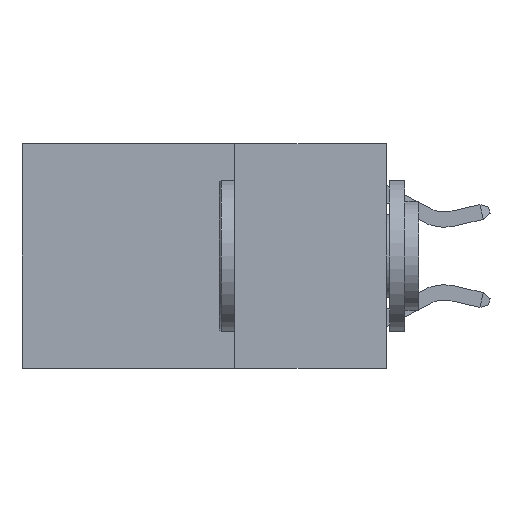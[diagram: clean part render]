
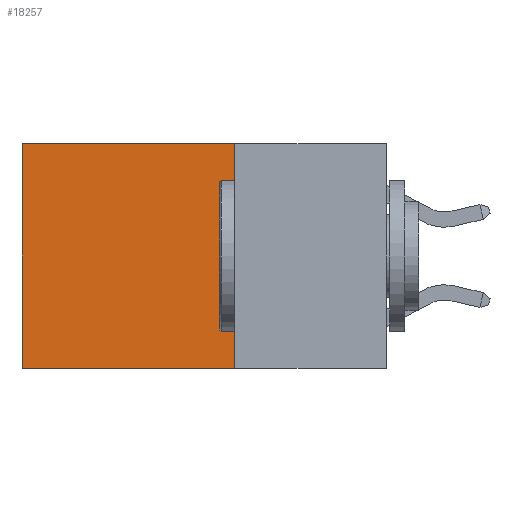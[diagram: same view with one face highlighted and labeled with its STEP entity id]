
A CAD part, left-side view. The second image highlights one B-rep face of the part: STEP entity #18257.
In plain terms, the highlighted planar face has unit normal (-1, 0, 0).
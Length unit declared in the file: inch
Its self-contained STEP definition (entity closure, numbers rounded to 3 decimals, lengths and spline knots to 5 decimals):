
#292 = CARTESIAN_POINT ( 'NONE',  ( 0.2625, 0.6, 0. ) ) ;
#810 = VERTEX_POINT ( 'NONE', #22380 ) ;
#1806 = EDGE_CURVE ( 'NONE', #18598, #12141, #10432, .T. ) ;
#2282 = LINE ( 'NONE', #292, #22768 ) ;
#3551 = DIRECTION ( 'NONE',  ( 0., 0., -1. ) ) ;
#5130 = VECTOR ( 'NONE', #16532, 39.37008 ) ;
#5199 = AXIS2_PLACEMENT_3D ( 'NONE', #7918, #26046, #3551 ) ;
#6414 = CARTESIAN_POINT ( 'NONE',  ( 0.2625, 0.6, -0.37 ) ) ;
#6752 = EDGE_CURVE ( 'NONE', #12141, #24361, #2282, .T. ) ;
#7513 = FACE_OUTER_BOUND ( 'NONE', #9814, .T. ) ;
#7712 = CARTESIAN_POINT ( 'NONE',  ( 0.2625, 0.25, 0. ) ) ;
#7918 = CARTESIAN_POINT ( 'NONE',  ( 0.2625, 0.25, 0. ) ) ;
#7941 = ORIENTED_EDGE ( 'NONE', *, *, #17400, .F. ) ;
#9814 = EDGE_LOOP ( 'NONE', ( #18756, #7941, #14336, #16081 ) ) ;
#10432 = LINE ( 'NONE', #12653, #19059 ) ;
#10559 = DIRECTION ( 'NONE',  ( 0., 1., 0. ) ) ;
#11722 = CARTESIAN_POINT ( 'NONE',  ( 0.2625, 0.25, 0. ) ) ;
#12141 = VERTEX_POINT ( 'NONE', #24973 ) ;
#12495 = VECTOR ( 'NONE', #13647, 39.37008 ) ;
#12570 = CARTESIAN_POINT ( 'NONE',  ( 0.2625, 0.25, -0.37 ) ) ;
#12653 = CARTESIAN_POINT ( 'NONE',  ( 0.2625, 0.25, 0. ) ) ;
#12789 = EDGE_CURVE ( 'NONE', #18598, #810, #16146, .T. ) ;
#13647 = DIRECTION ( 'NONE',  ( 0., 0., -1. ) ) ;
#14336 = ORIENTED_EDGE ( 'NONE', *, *, #12789, .F. ) ;
#16081 = ORIENTED_EDGE ( 'NONE', *, *, #1806, .T. ) ;
#16146 = LINE ( 'NONE', #7712, #12495 ) ;
#16532 = DIRECTION ( 'NONE',  ( 0., 1., 0. ) ) ;
#17400 = EDGE_CURVE ( 'NONE', #810, #24361, #24792, .T. ) ;
#18257 = ADVANCED_FACE ( 'NONE', ( #7513 ), #21669, .F. ) ;
#18598 = VERTEX_POINT ( 'NONE', #11722 ) ;
#18756 = ORIENTED_EDGE ( 'NONE', *, *, #6752, .T. ) ;
#19059 = VECTOR ( 'NONE', #10559, 39.37008 ) ;
#21669 = PLANE ( 'NONE',  #5199 ) ;
#22380 = CARTESIAN_POINT ( 'NONE',  ( 0.2625, 0.25, -0.37 ) ) ;
#22547 = DIRECTION ( 'NONE',  ( 0., 0., -1. ) ) ;
#22768 = VECTOR ( 'NONE', #22547, 39.37008 ) ;
#24361 = VERTEX_POINT ( 'NONE', #6414 ) ;
#24792 = LINE ( 'NONE', #12570, #5130 ) ;
#24973 = CARTESIAN_POINT ( 'NONE',  ( 0.2625, 0.6, 0. ) ) ;
#26046 = DIRECTION ( 'NONE',  ( 1., 0., 0. ) ) ;
